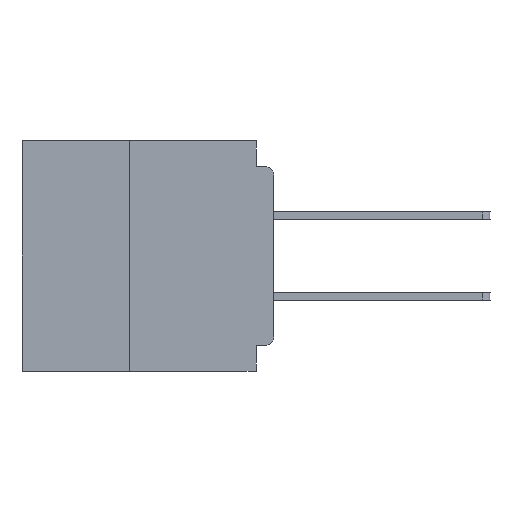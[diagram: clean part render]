
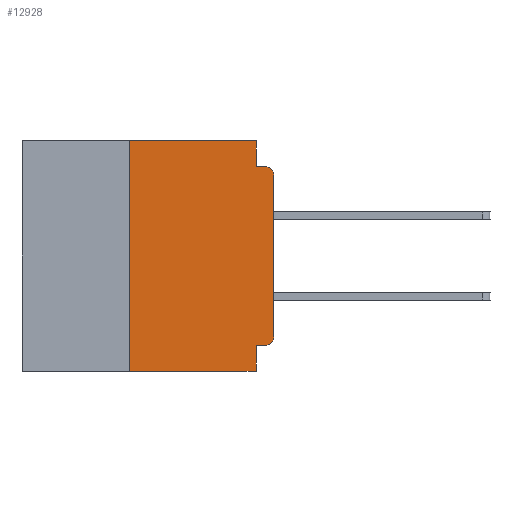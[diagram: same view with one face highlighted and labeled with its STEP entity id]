
A CAD part, left-side view. The second image highlights one B-rep face of the part: STEP entity #12928.
In plain terms, the highlighted planar face has unit normal (-1, 0, 0).
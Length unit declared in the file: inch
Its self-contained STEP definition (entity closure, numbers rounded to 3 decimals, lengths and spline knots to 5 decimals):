
#440 = CARTESIAN_POINT ( 'NONE',  ( 0., 0.015, -0.045 ) ) ;
#1233 = DIRECTION ( 'NONE',  ( 0., -1., 0. ) ) ;
#3068 = ORIENTED_EDGE ( 'NONE', *, *, #33935, .T. ) ;
#3354 = EDGE_CURVE ( 'NONE', #13585, #47219, #12955, .T. ) ;
#3879 = CARTESIAN_POINT ( 'NONE',  ( 0., 0.015, -0.355 ) ) ;
#5896 = DIRECTION ( 'NONE',  ( 0., 0., -1. ) ) ;
#6411 = LINE ( 'NONE', #51952, #20656 ) ;
#6532 = AXIS2_PLACEMENT_3D ( 'NONE', #22246, #55471, #27029 ) ;
#7407 = AXIS2_PLACEMENT_3D ( 'NONE', #39094, #34557, #5896 ) ;
#8400 = DIRECTION ( 'NONE',  ( 0., 0., -1. ) ) ;
#11474 = VERTEX_POINT ( 'NONE', #41731 ) ;
#12076 = LINE ( 'NONE', #30870, #40429 ) ;
#12313 = DIRECTION ( 'NONE',  ( 0., -1., 0. ) ) ;
#12928 = ADVANCED_FACE ( 'NONE', ( #35432 ), #24954, .F. ) ;
#12955 = LINE ( 'NONE', #22663, #49390 ) ;
#13585 = VERTEX_POINT ( 'NONE', #19887 ) ;
#16810 = EDGE_CURVE ( 'NONE', #45095, #47219, #24402, .T. ) ;
#17337 = ORIENTED_EDGE ( 'NONE', *, *, #61518, .F. ) ;
#17579 = EDGE_CURVE ( 'NONE', #50138, #13585, #31773, .T. ) ;
#18909 = LINE ( 'NONE', #49100, #56794 ) ;
#18946 = EDGE_CURVE ( 'NONE', #41175, #55881, #18909, .T. ) ;
#19887 = CARTESIAN_POINT ( 'NONE',  ( 0., 0.031, -0.355 ) ) ;
#20656 = VECTOR ( 'NONE', #23538, 39.37008 ) ;
#20679 = EDGE_CURVE ( 'NONE', #50138, #44459, #33852, .T. ) ;
#21033 = CARTESIAN_POINT ( 'NONE',  ( 0., 0.015, -0.34 ) ) ;
#21125 = DIRECTION ( 'NONE',  ( 0., -1., 0. ) ) ;
#21937 = CARTESIAN_POINT ( 'NONE',  ( 0., 0.437, -0.4 ) ) ;
#22246 = CARTESIAN_POINT ( 'NONE',  ( 0., 0.015, -0.06 ) ) ;
#22263 = ORIENTED_EDGE ( 'NONE', *, *, #55982, .F. ) ;
#22663 = CARTESIAN_POINT ( 'NONE',  ( 0., 0.031, -0.4 ) ) ;
#22769 = CARTESIAN_POINT ( 'NONE',  ( 0., 0.25, 0. ) ) ;
#22797 = CARTESIAN_POINT ( 'NONE',  ( 0., 0.031, -0.4 ) ) ;
#23276 = ORIENTED_EDGE ( 'NONE', *, *, #17579, .F. ) ;
#23538 = DIRECTION ( 'NONE',  ( 0., 0., -1. ) ) ;
#24402 = LINE ( 'NONE', #21937, #38563 ) ;
#24954 = PLANE ( 'NONE',  #7407 ) ;
#25005 = DIRECTION ( 'NONE',  ( 0., 1., 0. ) ) ;
#25489 = LINE ( 'NONE', #30700, #60405 ) ;
#25822 = DIRECTION ( 'NONE',  ( 0., 0., -1. ) ) ;
#26072 = DIRECTION ( 'NONE',  ( 0., 0., 1. ) ) ;
#26286 = ORIENTED_EDGE ( 'NONE', *, *, #36611, .T. ) ;
#27029 = DIRECTION ( 'NONE',  ( 0., 0., -1. ) ) ;
#29482 = CARTESIAN_POINT ( 'NONE',  ( 0., 0.031, -0.045 ) ) ;
#29793 = CARTESIAN_POINT ( 'NONE',  ( 0., 0., -0.355 ) ) ;
#30186 = CARTESIAN_POINT ( 'NONE',  ( 0., 0.25, -0.4 ) ) ;
#30700 = CARTESIAN_POINT ( 'NONE',  ( 0., 0.437, 0. ) ) ;
#30870 = CARTESIAN_POINT ( 'NONE',  ( 0., 0.25, -0.4 ) ) ;
#30973 = LINE ( 'NONE', #49525, #54734 ) ;
#31182 = CARTESIAN_POINT ( 'NONE',  ( 0., 0.031, 0. ) ) ;
#31773 = LINE ( 'NONE', #29793, #55504 ) ;
#33852 = CIRCLE ( 'NONE', #35871, 0.015 ) ;
#33935 = EDGE_CURVE ( 'NONE', #11474, #55881, #46054, .T. ) ;
#34557 = DIRECTION ( 'NONE',  ( 1., 0., 0. ) ) ;
#34908 = VERTEX_POINT ( 'NONE', #22769 ) ;
#35432 = FACE_OUTER_BOUND ( 'NONE', #45670, .T. ) ;
#35871 = AXIS2_PLACEMENT_3D ( 'NONE', #21033, #54251, #25822 ) ;
#36611 = EDGE_CURVE ( 'NONE', #44459, #11474, #30973, .T. ) ;
#38245 = VERTEX_POINT ( 'NONE', #31182 ) ;
#38563 = VECTOR ( 'NONE', #12313, 39.37008 ) ;
#39094 = CARTESIAN_POINT ( 'NONE',  ( 0., 0.437, 0. ) ) ;
#40429 = VECTOR ( 'NONE', #26072, 39.37008 ) ;
#41175 = VERTEX_POINT ( 'NONE', #29482 ) ;
#41731 = CARTESIAN_POINT ( 'NONE',  ( 0., 0., -0.06 ) ) ;
#42844 = ORIENTED_EDGE ( 'NONE', *, *, #18946, .F. ) ;
#44459 = VERTEX_POINT ( 'NONE', #58628 ) ;
#44765 = DIRECTION ( 'NONE',  ( 0., 0., 1. ) ) ;
#45095 = VERTEX_POINT ( 'NONE', #30186 ) ;
#45670 = EDGE_LOOP ( 'NONE', ( #26286, #3068, #42844, #17337, #22263, #53060, #51372, #55092, #23276, #59504 ) ) ;
#46054 = CIRCLE ( 'NONE', #6532, 0.015 ) ;
#47219 = VERTEX_POINT ( 'NONE', #22797 ) ;
#49100 = CARTESIAN_POINT ( 'NONE',  ( 0., 0., -0.045 ) ) ;
#49390 = VECTOR ( 'NONE', #8400, 39.37008 ) ;
#49525 = CARTESIAN_POINT ( 'NONE',  ( 0., 0., 0. ) ) ;
#50138 = VERTEX_POINT ( 'NONE', #3879 ) ;
#51372 = ORIENTED_EDGE ( 'NONE', *, *, #16810, .T. ) ;
#51952 = CARTESIAN_POINT ( 'NONE',  ( 0., 0.031, 0. ) ) ;
#53060 = ORIENTED_EDGE ( 'NONE', *, *, #58502, .F. ) ;
#54251 = DIRECTION ( 'NONE',  ( -1., 0., 0. ) ) ;
#54734 = VECTOR ( 'NONE', #44765, 39.37008 ) ;
#55092 = ORIENTED_EDGE ( 'NONE', *, *, #3354, .F. ) ;
#55471 = DIRECTION ( 'NONE',  ( -1., 0., 0. ) ) ;
#55504 = VECTOR ( 'NONE', #25005, 39.37008 ) ;
#55881 = VERTEX_POINT ( 'NONE', #440 ) ;
#55982 = EDGE_CURVE ( 'NONE', #34908, #38245, #25489, .T. ) ;
#56794 = VECTOR ( 'NONE', #1233, 39.37008 ) ;
#58502 = EDGE_CURVE ( 'NONE', #45095, #34908, #12076, .T. ) ;
#58628 = CARTESIAN_POINT ( 'NONE',  ( 0., 0., -0.34 ) ) ;
#59504 = ORIENTED_EDGE ( 'NONE', *, *, #20679, .T. ) ;
#60405 = VECTOR ( 'NONE', #21125, 39.37008 ) ;
#61518 = EDGE_CURVE ( 'NONE', #38245, #41175, #6411, .T. ) ;
